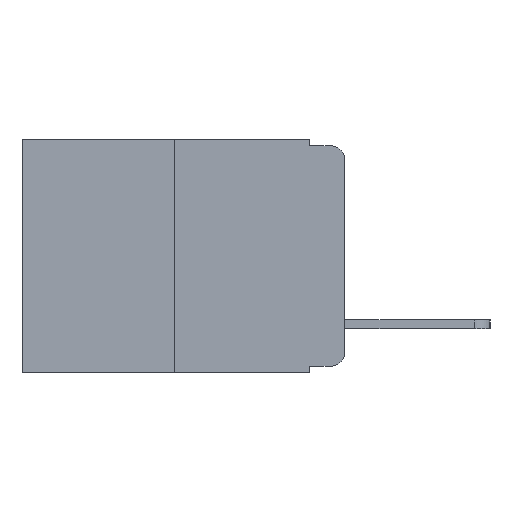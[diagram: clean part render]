
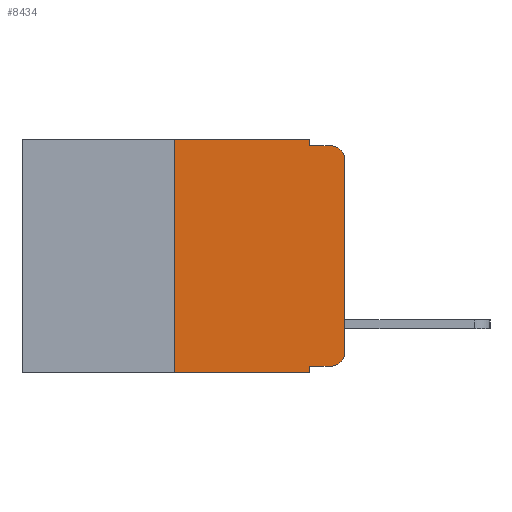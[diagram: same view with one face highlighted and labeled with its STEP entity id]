
A CAD part, left-side view. The second image highlights one B-rep face of the part: STEP entity #8434.
In plain terms, the highlighted planar face has unit normal (-1, 0, 0).
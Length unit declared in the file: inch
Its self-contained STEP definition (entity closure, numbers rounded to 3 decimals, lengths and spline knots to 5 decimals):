
#6 = VECTOR ( 'NONE', #1931, 39.37008 ) ;
#133 = EDGE_CURVE ( 'NONE', #17850, #2433, #226, .T. ) ;
#164 = CARTESIAN_POINT ( 'NONE',  ( 0., 0.051, 0. ) ) ;
#226 = LINE ( 'NONE', #13292, #11155 ) ;
#508 = EDGE_CURVE ( 'NONE', #11891, #12246, #10015, .T. ) ;
#509 = DIRECTION ( 'NONE',  ( 0., 0., -1. ) ) ;
#532 = EDGE_CURVE ( 'NONE', #15230, #12246, #13833, .T. ) ;
#538 = EDGE_CURVE ( 'NONE', #5703, #15230, #12918, .T. ) ;
#547 = LINE ( 'NONE', #6837, #6 ) ;
#1693 = EDGE_LOOP ( 'NONE', ( #6708, #16267, #4443, #16410, #3435, #5512, #2584, #13807, #15422, #14599 ) ) ;
#1860 = LINE ( 'NONE', #17316, #13525 ) ;
#1931 = DIRECTION ( 'NONE',  ( 0., -1., 0. ) ) ;
#2385 = AXIS2_PLACEMENT_3D ( 'NONE', #17729, #9426, #509 ) ;
#2433 = VERTEX_POINT ( 'NONE', #3864 ) ;
#2584 = ORIENTED_EDGE ( 'NONE', *, *, #4884, .T. ) ;
#2741 = VERTEX_POINT ( 'NONE', #2966 ) ;
#2966 = CARTESIAN_POINT ( 'NONE',  ( 0., 0.051, -0.343 ) ) ;
#3354 = VERTEX_POINT ( 'NONE', #15144 ) ;
#3435 = ORIENTED_EDGE ( 'NONE', *, *, #4750, .F. ) ;
#3442 = VERTEX_POINT ( 'NONE', #9151 ) ;
#3531 = CARTESIAN_POINT ( 'NONE',  ( 0., 0.051, -0.333 ) ) ;
#3654 = CARTESIAN_POINT ( 'NONE',  ( 0., 0.02, -0.03 ) ) ;
#3864 = CARTESIAN_POINT ( 'NONE',  ( 0., 0.02, -0.333 ) ) ;
#4443 = ORIENTED_EDGE ( 'NONE', *, *, #532, .F. ) ;
#4499 = CARTESIAN_POINT ( 'NONE',  ( 0., 0.473, 0. ) ) ;
#4712 = AXIS2_PLACEMENT_3D ( 'NONE', #4499, #18602, #10417 ) ;
#4750 = EDGE_CURVE ( 'NONE', #3442, #5703, #547, .T. ) ;
#4805 = DIRECTION ( 'NONE',  ( 0., 0., -1. ) ) ;
#4814 = CIRCLE ( 'NONE', #2385, 0.02 ) ;
#4884 = EDGE_CURVE ( 'NONE', #3354, #2741, #5673, .T. ) ;
#4994 = EDGE_CURVE ( 'NONE', #17850, #2741, #18059, .T. ) ;
#5199 = VECTOR ( 'NONE', #5928, 39.37008 ) ;
#5512 = ORIENTED_EDGE ( 'NONE', *, *, #15466, .F. ) ;
#5673 = LINE ( 'NONE', #18358, #16587 ) ;
#5703 = VERTEX_POINT ( 'NONE', #8865 ) ;
#5726 = AXIS2_PLACEMENT_3D ( 'NONE', #3654, #6479, #4805 ) ;
#5782 = CARTESIAN_POINT ( 'NONE',  ( 0., 0.25, 0. ) ) ;
#5928 = DIRECTION ( 'NONE',  ( 0., 0., -1. ) ) ;
#6437 = DIRECTION ( 'NONE',  ( 0., -1., 0. ) ) ;
#6479 = DIRECTION ( 'NONE',  ( -1., 0., 0. ) ) ;
#6631 = EDGE_CURVE ( 'NONE', #16020, #11891, #1860, .T. ) ;
#6708 = ORIENTED_EDGE ( 'NONE', *, *, #6631, .T. ) ;
#6727 = CARTESIAN_POINT ( 'NONE',  ( 0., 0.051, -0.01 ) ) ;
#6837 = CARTESIAN_POINT ( 'NONE',  ( 0., 0.473, 0. ) ) ;
#7238 = DIRECTION ( 'NONE',  ( 0., 0., 1. ) ) ;
#7734 = DIRECTION ( 'NONE',  ( 0., 0., -1. ) ) ;
#8213 = VECTOR ( 'NONE', #7238, 39.37008 ) ;
#8434 = ADVANCED_FACE ( 'NONE', ( #15386 ), #14560, .F. ) ;
#8702 = LINE ( 'NONE', #5782, #8213 ) ;
#8865 = CARTESIAN_POINT ( 'NONE',  ( 0., 0.051, 0. ) ) ;
#9151 = CARTESIAN_POINT ( 'NONE',  ( 0., 0.25, 0. ) ) ;
#9426 = DIRECTION ( 'NONE',  ( -1., 0., 0. ) ) ;
#10015 = CIRCLE ( 'NONE', #5726, 0.02 ) ;
#10417 = DIRECTION ( 'NONE',  ( 0., 0., -1. ) ) ;
#11155 = VECTOR ( 'NONE', #13442, 39.37008 ) ;
#11718 = CARTESIAN_POINT ( 'NONE',  ( 0., 0.051, -0.01 ) ) ;
#11891 = VERTEX_POINT ( 'NONE', #18156 ) ;
#12246 = VERTEX_POINT ( 'NONE', #16257 ) ;
#12918 = LINE ( 'NONE', #164, #5199 ) ;
#13216 = DIRECTION ( 'NONE',  ( 0., -1., 0. ) ) ;
#13292 = CARTESIAN_POINT ( 'NONE',  ( 0., 0.051, -0.333 ) ) ;
#13352 = VECTOR ( 'NONE', #6437, 39.37008 ) ;
#13442 = DIRECTION ( 'NONE',  ( 0., -1., 0. ) ) ;
#13525 = VECTOR ( 'NONE', #16994, 39.37008 ) ;
#13807 = ORIENTED_EDGE ( 'NONE', *, *, #4994, .F. ) ;
#13833 = LINE ( 'NONE', #11718, #13352 ) ;
#14502 = VECTOR ( 'NONE', #7734, 39.37008 ) ;
#14560 = PLANE ( 'NONE',  #4712 ) ;
#14599 = ORIENTED_EDGE ( 'NONE', *, *, #14901, .T. ) ;
#14901 = EDGE_CURVE ( 'NONE', #2433, #16020, #4814, .T. ) ;
#15144 = CARTESIAN_POINT ( 'NONE',  ( 0., 0.25, -0.343 ) ) ;
#15230 = VERTEX_POINT ( 'NONE', #6727 ) ;
#15386 = FACE_OUTER_BOUND ( 'NONE', #1693, .T. ) ;
#15422 = ORIENTED_EDGE ( 'NONE', *, *, #133, .T. ) ;
#15466 = EDGE_CURVE ( 'NONE', #3354, #3442, #8702, .T. ) ;
#16020 = VERTEX_POINT ( 'NONE', #17000 ) ;
#16257 = CARTESIAN_POINT ( 'NONE',  ( 0., 0.02, -0.01 ) ) ;
#16267 = ORIENTED_EDGE ( 'NONE', *, *, #508, .T. ) ;
#16410 = ORIENTED_EDGE ( 'NONE', *, *, #538, .F. ) ;
#16587 = VECTOR ( 'NONE', #13216, 39.37008 ) ;
#16891 = CARTESIAN_POINT ( 'NONE',  ( 0., 0.051, 0. ) ) ;
#16994 = DIRECTION ( 'NONE',  ( 0., 0., 1. ) ) ;
#17000 = CARTESIAN_POINT ( 'NONE',  ( 0., 0., -0.313 ) ) ;
#17316 = CARTESIAN_POINT ( 'NONE',  ( 0., 0., 0. ) ) ;
#17729 = CARTESIAN_POINT ( 'NONE',  ( 0., 0.02, -0.313 ) ) ;
#17850 = VERTEX_POINT ( 'NONE', #3531 ) ;
#18059 = LINE ( 'NONE', #16891, #14502 ) ;
#18156 = CARTESIAN_POINT ( 'NONE',  ( 0., 0., -0.03 ) ) ;
#18358 = CARTESIAN_POINT ( 'NONE',  ( 0., 0.473, -0.343 ) ) ;
#18602 = DIRECTION ( 'NONE',  ( 1., 0., 0. ) ) ;
